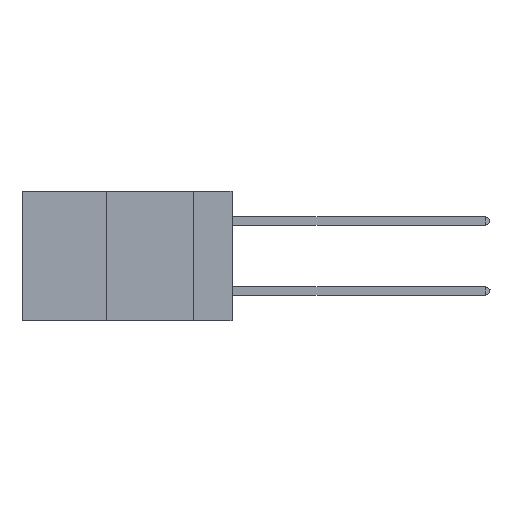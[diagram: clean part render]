
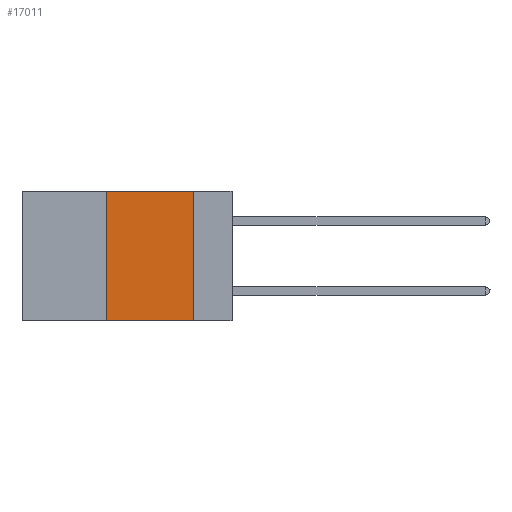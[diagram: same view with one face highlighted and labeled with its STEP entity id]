
A CAD part, left-side view. The second image highlights one B-rep face of the part: STEP entity #17011.
In plain terms, the highlighted planar face has unit normal (-1, 0, 0).
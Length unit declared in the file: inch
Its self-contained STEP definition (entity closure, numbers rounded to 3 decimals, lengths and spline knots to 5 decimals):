
#884 = VECTOR ( 'NONE', #4014, 39.37008 ) ;
#1490 = VERTEX_POINT ( 'NONE', #8303 ) ;
#1751 = FACE_OUTER_BOUND ( 'NONE', #10598, .T. ) ;
#2075 = CARTESIAN_POINT ( 'NONE',  ( 0., 0.6, 0. ) ) ;
#2111 = DIRECTION ( 'NONE',  ( 0., 0., -1. ) ) ;
#2662 = VECTOR ( 'NONE', #15134, 39.37008 ) ;
#4014 = DIRECTION ( 'NONE',  ( 0., -1., 0. ) ) ;
#4045 = EDGE_CURVE ( 'NONE', #11391, #22364, #11318, .T. ) ;
#5749 = CARTESIAN_POINT ( 'NONE',  ( 0., 0.6, 0. ) ) ;
#8303 = CARTESIAN_POINT ( 'NONE',  ( 0., 0.36, 0. ) ) ;
#8468 = VERTEX_POINT ( 'NONE', #14173 ) ;
#8487 = LINE ( 'NONE', #12368, #2662 ) ;
#8831 = ORIENTED_EDGE ( 'NONE', *, *, #4045, .F. ) ;
#10598 = EDGE_LOOP ( 'NONE', ( #8831, #14174, #13079, #20940 ) ) ;
#10970 = CARTESIAN_POINT ( 'NONE',  ( 0., 0.11, -0.37 ) ) ;
#11318 = LINE ( 'NONE', #20905, #23703 ) ;
#11391 = VERTEX_POINT ( 'NONE', #12089 ) ;
#12089 = CARTESIAN_POINT ( 'NONE',  ( 0., 0.11, 0. ) ) ;
#12368 = CARTESIAN_POINT ( 'NONE',  ( 0., 0.6, -0.37 ) ) ;
#13079 = ORIENTED_EDGE ( 'NONE', *, *, #16219, .F. ) ;
#13129 = PLANE ( 'NONE',  #22730 ) ;
#14173 = CARTESIAN_POINT ( 'NONE',  ( 0., 0.36, -0.37 ) ) ;
#14174 = ORIENTED_EDGE ( 'NONE', *, *, #16072, .F. ) ;
#14387 = DIRECTION ( 'NONE',  ( 0., 0., 1. ) ) ;
#15134 = DIRECTION ( 'NONE',  ( 0., -1., 0. ) ) ;
#15513 = DIRECTION ( 'NONE',  ( 0., 0., -1. ) ) ;
#16072 = EDGE_CURVE ( 'NONE', #1490, #11391, #19731, .T. ) ;
#16204 = EDGE_CURVE ( 'NONE', #8468, #22364, #8487, .T. ) ;
#16219 = EDGE_CURVE ( 'NONE', #8468, #1490, #20295, .T. ) ;
#16809 = CARTESIAN_POINT ( 'NONE',  ( 0., 0.36, 0. ) ) ;
#17011 = ADVANCED_FACE ( 'NONE', ( #1751 ), #13129, .F. ) ;
#18708 = DIRECTION ( 'NONE',  ( 1., 0., 0. ) ) ;
#19731 = LINE ( 'NONE', #2075, #884 ) ;
#20295 = LINE ( 'NONE', #16809, #22553 ) ;
#20905 = CARTESIAN_POINT ( 'NONE',  ( 0., 0.11, 0. ) ) ;
#20940 = ORIENTED_EDGE ( 'NONE', *, *, #16204, .T. ) ;
#22364 = VERTEX_POINT ( 'NONE', #10970 ) ;
#22553 = VECTOR ( 'NONE', #14387, 39.37008 ) ;
#22730 = AXIS2_PLACEMENT_3D ( 'NONE', #5749, #18708, #2111 ) ;
#23703 = VECTOR ( 'NONE', #15513, 39.37008 ) ;
